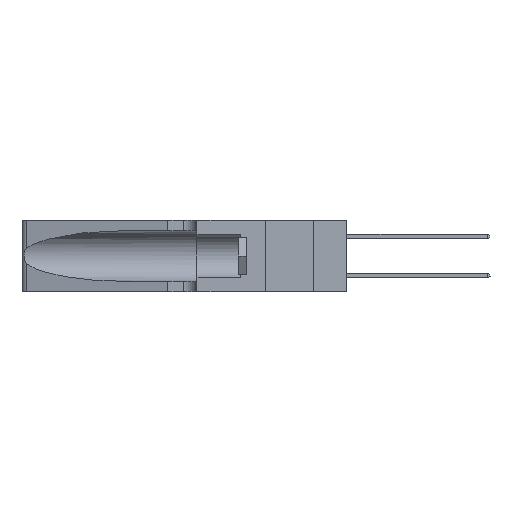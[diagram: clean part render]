
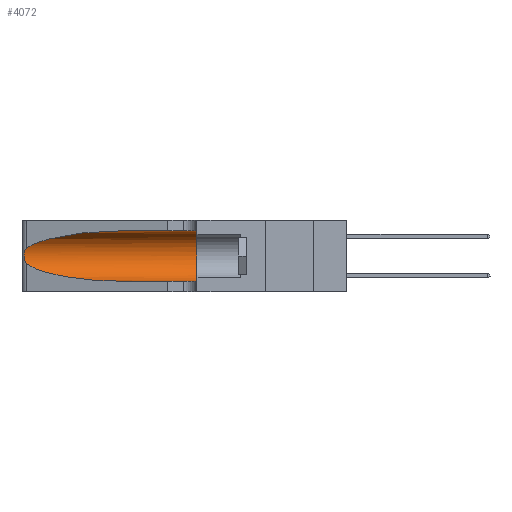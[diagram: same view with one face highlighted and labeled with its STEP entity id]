
A CAD part, left-side view. The second image highlights one B-rep face of the part: STEP entity #4072.
In plain terms, the highlighted cylindrical face has radius 3.308 mm (diameter 6.617 mm), a partial arc.
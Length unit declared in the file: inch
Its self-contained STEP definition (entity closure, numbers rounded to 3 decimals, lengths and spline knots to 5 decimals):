
#77 = ORIENTED_EDGE ( 'NONE', *, *, #421, .F. ) ;
#232 = ORIENTED_EDGE ( 'NONE', *, *, #33571, .F. ) ;
#421 = EDGE_CURVE ( 'NONE', #19511, #5659, #14760, .T. ) ;
#1219 = CARTESIAN_POINT ( 'NONE',  ( 0.25555, 1.22993, 0.14849 ) ) ;
#3898 = CARTESIAN_POINT ( 'NONE',  ( 0.25856, 1.23593, 0.16098 ) ) ;
#4072 = ADVANCED_FACE ( 'NONE', ( #23136 ), #17350, .F. ) ;
#4299 = CARTESIAN_POINT ( 'NONE',  ( 0.1305, 0.72297, 0.31525 ) ) ;
#4433 = CARTESIAN_POINT ( 'NONE',  ( 0.1305, 0.72297, 0.05475 ) ) ;
#4741 = VERTEX_POINT ( 'NONE', #16969 ) ;
#5659 = VERTEX_POINT ( 'NONE', #24030 ) ;
#6176 = AXIS2_PLACEMENT_3D ( 'NONE', #14924, #30835, #33461 ) ;
#6194 = CARTESIAN_POINT ( 'NONE',  ( 0.25487, 1.22718, 0.22369 ) ) ;
#6256 = CARTESIAN_POINT ( 'NONE',  ( 0.1305, 0.72297, 0.05475 ) ) ;
#7201 = CARTESIAN_POINT ( 'NONE',  ( 0.18966, 0.96281, 0.05475 ) ) ;
#7282 = CARTESIAN_POINT ( 'NONE',  ( 0.1305, 1.61858, 0.185 ) ) ;
#7781 = CARTESIAN_POINT ( 'NONE',  ( 0.25487, 1.22718, 0.14631 ) ) ;
#9030 = CARTESIAN_POINT ( 'NONE',  ( 0.25487, 1.22718, 0.14631 ) ) ;
#9155 = CARTESIAN_POINT ( 'NONE',  ( 0.25639, 1.23184, 0.21858 ) ) ;
#10086 = CARTESIAN_POINT ( 'NONE',  ( 0.25487, 1.22718, 0.14631 ) ) ;
#10158 = CARTESIAN_POINT ( 'NONE',  ( 0.18966, 0.96281, 0.31525 ) ) ;
#10372 = VECTOR ( 'NONE', #25083, 39.37008 ) ;
#11393 = CARTESIAN_POINT ( 'NONE',  ( 0.25789, 1.23486, 0.15765 ) ) ;
#11938 = LINE ( 'NONE', #13884, #10372 ) ;
#12305 = VERTEX_POINT ( 'NONE', #4299 ) ;
#12628 = CARTESIAN_POINT ( 'NONE',  ( 0.1305, 0.72297, 0.31525 ) ) ;
#12773 = AXIS2_PLACEMENT_3D ( 'NONE', #7282, #17568, #14839 ) ;
#13884 = CARTESIAN_POINT ( 'NONE',  ( 0.1305, 1.61858, 0.05475 ) ) ;
#14121 = CARTESIAN_POINT ( 'NONE',  ( 0.25555, 1.22994, 0.2215 ) ) ;
#14760 = CIRCLE ( 'NONE', #6176, 0.13025 ) ;
#14839 = DIRECTION ( 'NONE',  ( 0., 0., -1. ) ) ;
#14924 = CARTESIAN_POINT ( 'NONE',  ( 0.1305, 0.35, 0.185 ) ) ;
#15312 = VERTEX_POINT ( 'NONE', #6256 ) ;
#16969 = CARTESIAN_POINT ( 'NONE',  ( 0.25487, 1.22718, 0.22369 ) ) ;
#17350 = CYLINDRICAL_SURFACE ( 'NONE', #12773, 0.13025 ) ;
#17568 = DIRECTION ( 'NONE',  ( 0., -1., 0. ) ) ;
#18287 = CARTESIAN_POINT ( 'NONE',  ( 0.1305, 1.61858, 0.31525 ) ) ;
#18852 = CARTESIAN_POINT ( 'NONE',  ( 0.1305, 0.35, 0.31525 ) ) ;
#19178 = EDGE_CURVE ( 'NONE', #29537, #15312, #32330, .T. ) ;
#19335 = CARTESIAN_POINT ( 'NONE',  ( 0.26075, 1.23896, 0.178 ) ) ;
#19511 = VERTEX_POINT ( 'NONE', #18852 ) ;
#19647 = EDGE_CURVE ( 'NONE', #12305, #4741, #27296, .T. ) ;
#20210 = B_SPLINE_CURVE_WITH_KNOTS ( 'NONE', 3,
 ( #6194, #14121, #9155, #29884, #24841, #22218, #29638, #19335, #24596, #3898, #11393, #22097, #1219, #9030 ),
 .UNSPECIFIED., .F., .F.,
 ( 4, 2, 2, 2, 2, 2, 4 ),
 ( 0., 0.00027, 0.00053, 0.00107, 0.0016, 0.00187, 0.00214 ),
 .UNSPECIFIED. ) ;
#21723 = EDGE_CURVE ( 'NONE', #15312, #5659, #11938, .T. ) ;
#22097 = CARTESIAN_POINT ( 'NONE',  ( 0.25639, 1.23186, 0.15144 ) ) ;
#22218 = CARTESIAN_POINT ( 'NONE',  ( 0.26018, 1.23835, 0.19895 ) ) ;
#23096 = CARTESIAN_POINT ( 'NONE',  ( 0.25487, 1.22718, 0.22369 ) ) ;
#23136 = FACE_OUTER_BOUND ( 'NONE', #26084, .T. ) ;
#23687 = EDGE_CURVE ( 'NONE', #4741, #29537, #20210, .T. ) ;
#24030 = CARTESIAN_POINT ( 'NONE',  ( 0.1305, 0.35, 0.05475 ) ) ;
#24596 = CARTESIAN_POINT ( 'NONE',  ( 0.26017, 1.23833, 0.17102 ) ) ;
#24841 = CARTESIAN_POINT ( 'NONE',  ( 0.25854, 1.2359, 0.20912 ) ) ;
#24871 = ORIENTED_EDGE ( 'NONE', *, *, #19178, .T. ) ;
#25083 = DIRECTION ( 'NONE',  ( 0., -1., 0. ) ) ;
#25191 = LINE ( 'NONE', #18287, #26794 ) ;
#26084 = EDGE_LOOP ( 'NONE', ( #30297, #33052, #24871, #30789, #77, #232 ) ) ;
#26794 = VECTOR ( 'NONE', #33642, 39.37008 ) ;
#27296 =( BOUNDED_CURVE ( )  B_SPLINE_CURVE ( 3, ( #12628, #10158, #33538, #23096 ),
 .UNSPECIFIED., .F., .F. ) 
 B_SPLINE_CURVE_WITH_KNOTS ( ( 4, 4 ),
 ( 1.5708, 2.84003 ),
 .UNSPECIFIED. ) 
 CURVE ( )  GEOMETRIC_REPRESENTATION_ITEM ( )  RATIONAL_B_SPLINE_CURVE ( ( 1., 0.87, 0.87, 1. ) ) 
 REPRESENTATION_ITEM ( '' )  );
#29537 = VERTEX_POINT ( 'NONE', #7781 ) ;
#29638 = CARTESIAN_POINT ( 'NONE',  ( 0.26075, 1.23896, 0.19203 ) ) ;
#29884 = CARTESIAN_POINT ( 'NONE',  ( 0.25787, 1.23484, 0.2124 ) ) ;
#30297 = ORIENTED_EDGE ( 'NONE', *, *, #19647, .T. ) ;
#30673 = CARTESIAN_POINT ( 'NONE',  ( 0.2373, 1.15595, 0.08982 ) ) ;
#30789 = ORIENTED_EDGE ( 'NONE', *, *, #21723, .T. ) ;
#30835 = DIRECTION ( 'NONE',  ( 0., 1., 0. ) ) ;
#32330 =( BOUNDED_CURVE ( )  B_SPLINE_CURVE ( 3, ( #10086, #30673, #7201, #4433 ),
 .UNSPECIFIED., .F., .T. ) 
 B_SPLINE_CURVE_WITH_KNOTS ( ( 4, 4 ),
 ( 3.44316, 4.71239 ),
 .UNSPECIFIED. ) 
 CURVE ( )  GEOMETRIC_REPRESENTATION_ITEM ( )  RATIONAL_B_SPLINE_CURVE ( ( 1., 0.87, 0.87, 1. ) ) 
 REPRESENTATION_ITEM ( '' )  );
#33052 = ORIENTED_EDGE ( 'NONE', *, *, #23687, .T. ) ;
#33461 = DIRECTION ( 'NONE',  ( 0., 0., 1. ) ) ;
#33538 = CARTESIAN_POINT ( 'NONE',  ( 0.2373, 1.15595, 0.28018 ) ) ;
#33571 = EDGE_CURVE ( 'NONE', #12305, #19511, #25191, .T. ) ;
#33642 = DIRECTION ( 'NONE',  ( 0., -1., 0. ) ) ;
